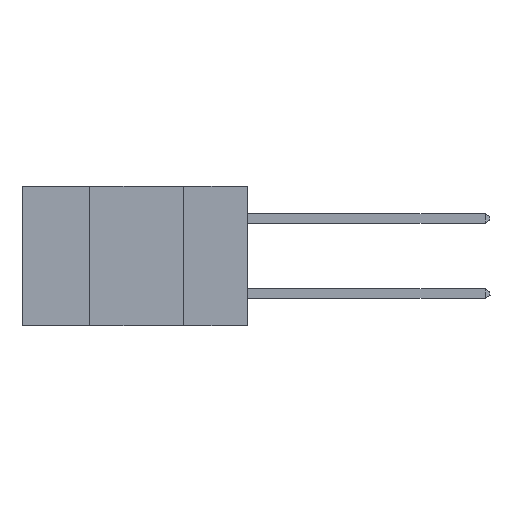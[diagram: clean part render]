
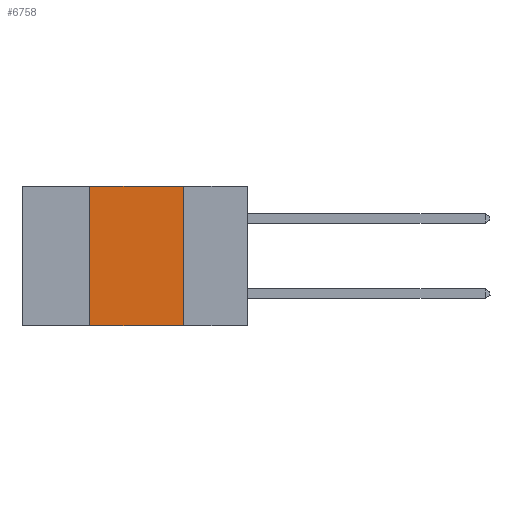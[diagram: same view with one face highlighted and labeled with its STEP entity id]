
A CAD part, left-side view. The second image highlights one B-rep face of the part: STEP entity #6758.
In plain terms, the highlighted planar face has unit normal (-1, 0, 0).
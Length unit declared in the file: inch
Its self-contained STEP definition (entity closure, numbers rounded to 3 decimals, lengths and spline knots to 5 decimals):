
#885 = CARTESIAN_POINT ( 'NONE',  ( 0., 0.6, -0.37 ) ) ;
#3817 = DIRECTION ( 'NONE',  ( 0., -1., 0. ) ) ;
#4221 = CARTESIAN_POINT ( 'NONE',  ( 0., 0.17, 0. ) ) ;
#5481 = VERTEX_POINT ( 'NONE', #27199 ) ;
#6758 = ADVANCED_FACE ( 'NONE', ( #26296 ), #19458, .F. ) ;
#6868 = CARTESIAN_POINT ( 'NONE',  ( 0., 0.42, 0. ) ) ;
#6953 = EDGE_LOOP ( 'NONE', ( #18096, #13843, #22968, #10473 ) ) ;
#7658 = CARTESIAN_POINT ( 'NONE',  ( 0., 0.17, -0.37 ) ) ;
#9526 = DIRECTION ( 'NONE',  ( 1., 0., 0. ) ) ;
#9537 = EDGE_CURVE ( 'NONE', #28127, #19680, #25730, .T. ) ;
#10473 = ORIENTED_EDGE ( 'NONE', *, *, #17952, .T. ) ;
#11338 = VECTOR ( 'NONE', #3817, 39.37008 ) ;
#12708 = LINE ( 'NONE', #6868, #31655 ) ;
#13843 = ORIENTED_EDGE ( 'NONE', *, *, #20019, .F. ) ;
#15812 = DIRECTION ( 'NONE',  ( 0., -1., 0. ) ) ;
#17952 = EDGE_CURVE ( 'NONE', #24654, #19680, #20873, .T. ) ;
#18096 = ORIENTED_EDGE ( 'NONE', *, *, #9537, .F. ) ;
#19458 = PLANE ( 'NONE',  #20015 ) ;
#19680 = VERTEX_POINT ( 'NONE', #7658 ) ;
#20015 = AXIS2_PLACEMENT_3D ( 'NONE', #24458, #9526, #26911 ) ;
#20019 = EDGE_CURVE ( 'NONE', #5481, #28127, #24603, .T. ) ;
#20873 = LINE ( 'NONE', #885, #27415 ) ;
#22968 = ORIENTED_EDGE ( 'NONE', *, *, #29500, .F. ) ;
#24198 = CARTESIAN_POINT ( 'NONE',  ( 0., 0.42, -0.37 ) ) ;
#24314 = DIRECTION ( 'NONE',  ( 0., 0., 1. ) ) ;
#24458 = CARTESIAN_POINT ( 'NONE',  ( 0., 0.6, 0. ) ) ;
#24603 = LINE ( 'NONE', #26226, #11338 ) ;
#24654 = VERTEX_POINT ( 'NONE', #24198 ) ;
#24970 = VECTOR ( 'NONE', #29476, 39.37008 ) ;
#25730 = LINE ( 'NONE', #27046, #24970 ) ;
#26226 = CARTESIAN_POINT ( 'NONE',  ( 0., 0.6, 0. ) ) ;
#26296 = FACE_OUTER_BOUND ( 'NONE', #6953, .T. ) ;
#26911 = DIRECTION ( 'NONE',  ( 0., 0., -1. ) ) ;
#27046 = CARTESIAN_POINT ( 'NONE',  ( 0., 0.17, 0. ) ) ;
#27199 = CARTESIAN_POINT ( 'NONE',  ( 0., 0.42, 0. ) ) ;
#27415 = VECTOR ( 'NONE', #15812, 39.37008 ) ;
#28127 = VERTEX_POINT ( 'NONE', #4221 ) ;
#29476 = DIRECTION ( 'NONE',  ( 0., 0., -1. ) ) ;
#29500 = EDGE_CURVE ( 'NONE', #24654, #5481, #12708, .T. ) ;
#31655 = VECTOR ( 'NONE', #24314, 39.37008 ) ;
